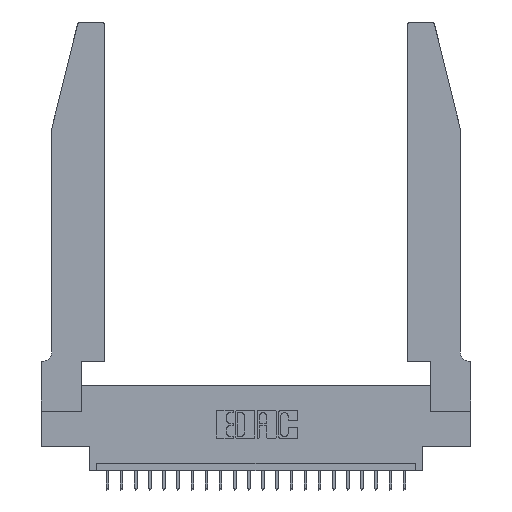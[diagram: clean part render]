
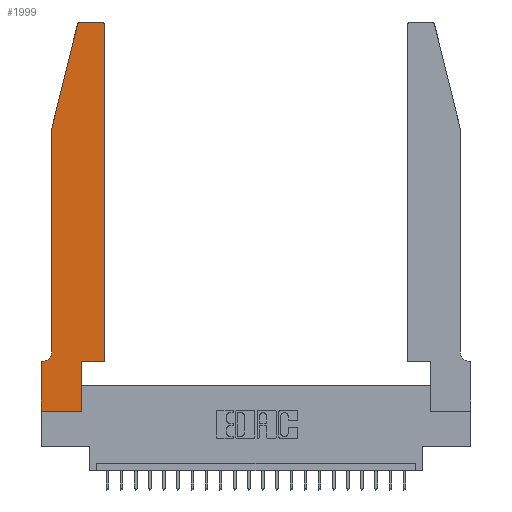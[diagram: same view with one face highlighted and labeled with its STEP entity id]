
A CAD part, top view. The second image highlights one B-rep face of the part: STEP entity #1999.
In plain terms, the highlighted planar face has unit normal (0, 0, 1).
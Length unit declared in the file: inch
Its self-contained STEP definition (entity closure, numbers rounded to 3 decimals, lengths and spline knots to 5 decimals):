
#53 = EDGE_CURVE ( 'NONE', #19041, #15948, #1308, .T. ) ;
#286 = ORIENTED_EDGE ( 'NONE', *, *, #4977, .T. ) ;
#426 = DIRECTION ( 'NONE',  ( -0.239, -0.971, 0. ) ) ;
#680 = ORIENTED_EDGE ( 'NONE', *, *, #19117, .T. ) ;
#777 = VECTOR ( 'NONE', #14901, 39.37008 ) ;
#782 = AXIS2_PLACEMENT_3D ( 'NONE', #13090, #3987, #14873 ) ;
#1308 = LINE ( 'NONE', #12774, #8461 ) ;
#1507 = ORIENTED_EDGE ( 'NONE', *, *, #4886, .T. ) ;
#1548 = VERTEX_POINT ( 'NONE', #2084 ) ;
#1744 = DIRECTION ( 'NONE',  ( 0., -1., 0. ) ) ;
#1999 = ADVANCED_FACE ( 'NONE', ( #22754 ), #20563, .T. ) ;
#2084 = CARTESIAN_POINT ( 'NONE',  ( 0.0755, 0.42, 0.37 ) ) ;
#2212 = EDGE_CURVE ( 'NONE', #3683, #22415, #21882, .T. ) ;
#2491 = DIRECTION ( 'NONE',  ( -1., 0., 0. ) ) ;
#2738 = EDGE_CURVE ( 'NONE', #4874, #9804, #19189, .T. ) ;
#3295 = CARTESIAN_POINT ( 'NONE',  ( 0.4205, 2.75, 0.37 ) ) ;
#3527 = CARTESIAN_POINT ( 'NONE',  ( 0., 0.35, 0.37 ) ) ;
#3683 = VERTEX_POINT ( 'NONE', #18636 ) ;
#3987 = DIRECTION ( 'NONE',  ( 0., 0., 1. ) ) ;
#4352 = CARTESIAN_POINT ( 'NONE',  ( 0.4505, 0.35, 0.37 ) ) ;
#4536 = CIRCLE ( 'NONE', #10803, 0.03 ) ;
#4874 = VERTEX_POINT ( 'NONE', #17412 ) ;
#4886 = EDGE_CURVE ( 'NONE', #22457, #3683, #23874, .T. ) ;
#4977 = EDGE_CURVE ( 'NONE', #16996, #4874, #4536, .T. ) ;
#5588 = CARTESIAN_POINT ( 'NONE',  ( 0., 0., 0.37 ) ) ;
#5748 = CARTESIAN_POINT ( 'NONE',  ( 0.0055, 0.42, 0.37 ) ) ;
#6837 = VERTEX_POINT ( 'NONE', #9846 ) ;
#7290 = CARTESIAN_POINT ( 'NONE',  ( 0., 0., 0.37 ) ) ;
#7775 = EDGE_CURVE ( 'NONE', #23308, #16996, #15610, .T. ) ;
#8461 = VECTOR ( 'NONE', #10922, 39.37008 ) ;
#8566 = CARTESIAN_POINT ( 'NONE',  ( 0., 0.35, 0.37 ) ) ;
#8638 = EDGE_CURVE ( 'NONE', #9804, #1548, #14750, .T. ) ;
#9295 = DIRECTION ( 'NONE',  ( 0., -1., 0. ) ) ;
#9340 = ORIENTED_EDGE ( 'NONE', *, *, #14296, .T. ) ;
#9355 = DIRECTION ( 'NONE',  ( -1., 0., 0. ) ) ;
#9476 = DIRECTION ( 'NONE',  ( 1., 0., 0. ) ) ;
#9804 = VERTEX_POINT ( 'NONE', #13866 ) ;
#9846 = CARTESIAN_POINT ( 'NONE',  ( 0.4505, 2.72, 0.37 ) ) ;
#10591 = DIRECTION ( 'NONE',  ( 0., 1., 0. ) ) ;
#10730 = ORIENTED_EDGE ( 'NONE', *, *, #16136, .T. ) ;
#10803 = AXIS2_PLACEMENT_3D ( 'NONE', #20234, #22051, #9476 ) ;
#10891 = CARTESIAN_POINT ( 'NONE',  ( 0.4505, 0.35, 0.37 ) ) ;
#10922 = DIRECTION ( 'NONE',  ( -1., 0., 0. ) ) ;
#11099 = CARTESIAN_POINT ( 'NONE',  ( 0.2865, 0., 0.37 ) ) ;
#11759 = CARTESIAN_POINT ( 'NONE',  ( 0.0755, 2., 0.37 ) ) ;
#11798 = CIRCLE ( 'NONE', #782, 0.03 ) ;
#11854 = DIRECTION ( 'NONE',  ( 0., 1., 0. ) ) ;
#12710 = CARTESIAN_POINT ( 'NONE',  ( 0.4505, 0.35, 0.37 ) ) ;
#12736 = VECTOR ( 'NONE', #11854, 39.37008 ) ;
#12774 = CARTESIAN_POINT ( 'NONE',  ( 0.0755, 0.35, 0.37 ) ) ;
#12817 = VECTOR ( 'NONE', #1744, 39.37008 ) ;
#13029 = DIRECTION ( 'NONE',  ( 0., 0., -1. ) ) ;
#13090 = CARTESIAN_POINT ( 'NONE',  ( 0.4205, 2.72, 0.37 ) ) ;
#13116 = CARTESIAN_POINT ( 'NONE',  ( 0., 0., 0.37 ) ) ;
#13446 = CARTESIAN_POINT ( 'NONE',  ( 0.284, 2.75, 0.37 ) ) ;
#13663 = ORIENTED_EDGE ( 'NONE', *, *, #53, .T. ) ;
#13866 = CARTESIAN_POINT ( 'NONE',  ( 0.0755, 2., 0.37 ) ) ;
#14010 = CARTESIAN_POINT ( 'NONE',  ( 0.2865, 0.35, 0.37 ) ) ;
#14296 = EDGE_CURVE ( 'NONE', #1548, #19041, #17600, .T. ) ;
#14462 = ORIENTED_EDGE ( 'NONE', *, *, #8638, .T. ) ;
#14750 = LINE ( 'NONE', #18526, #12817 ) ;
#14821 = EDGE_CURVE ( 'NONE', #6837, #23308, #11798, .T. ) ;
#14870 = VECTOR ( 'NONE', #9295, 39.37008 ) ;
#14873 = DIRECTION ( 'NONE',  ( 1., 0., 0. ) ) ;
#14901 = DIRECTION ( 'NONE',  ( 1., 0., 0. ) ) ;
#14988 = ORIENTED_EDGE ( 'NONE', *, *, #23970, .T. ) ;
#15597 = VERTEX_POINT ( 'NONE', #5588 ) ;
#15604 = LINE ( 'NONE', #4352, #12736 ) ;
#15610 = LINE ( 'NONE', #17315, #17453 ) ;
#15948 = VERTEX_POINT ( 'NONE', #8566 ) ;
#16100 = ORIENTED_EDGE ( 'NONE', *, *, #14821, .T. ) ;
#16136 = EDGE_CURVE ( 'NONE', #15948, #15597, #24059, .T. ) ;
#16996 = VERTEX_POINT ( 'NONE', #13446 ) ;
#17315 = CARTESIAN_POINT ( 'NONE',  ( 0.2605, 2.75, 0.37 ) ) ;
#17412 = CARTESIAN_POINT ( 'NONE',  ( 0.25487, 2.72718, 0.37 ) ) ;
#17453 = VECTOR ( 'NONE', #2491, 39.37008 ) ;
#17600 = CIRCLE ( 'NONE', #22682, 0.07 ) ;
#18313 = DIRECTION ( 'NONE',  ( 1., 0., 0. ) ) ;
#18517 = AXIS2_PLACEMENT_3D ( 'NONE', #3527, #22511, #18833 ) ;
#18526 = CARTESIAN_POINT ( 'NONE',  ( 0.0755, 2., 0.37 ) ) ;
#18537 = VECTOR ( 'NONE', #10591, 39.37008 ) ;
#18611 = ORIENTED_EDGE ( 'NONE', *, *, #2738, .T. ) ;
#18636 = CARTESIAN_POINT ( 'NONE',  ( 0.2865, 0.35, 0.37 ) ) ;
#18833 = DIRECTION ( 'NONE',  ( 1., 0., 0. ) ) ;
#19041 = VERTEX_POINT ( 'NONE', #21793 ) ;
#19117 = EDGE_CURVE ( 'NONE', #15597, #22457, #20796, .T. ) ;
#19189 = LINE ( 'NONE', #11759, #20356 ) ;
#19518 = ORIENTED_EDGE ( 'NONE', *, *, #7775, .T. ) ;
#20234 = CARTESIAN_POINT ( 'NONE',  ( 0.284, 2.72, 0.37 ) ) ;
#20356 = VECTOR ( 'NONE', #426, 39.37008 ) ;
#20563 = PLANE ( 'NONE',  #18517 ) ;
#20796 = LINE ( 'NONE', #13116, #777 ) ;
#21793 = CARTESIAN_POINT ( 'NONE',  ( 0.0055, 0.35, 0.37 ) ) ;
#21882 = LINE ( 'NONE', #10891, #23907 ) ;
#22051 = DIRECTION ( 'NONE',  ( 0., 0., 1. ) ) ;
#22415 = VERTEX_POINT ( 'NONE', #12710 ) ;
#22457 = VERTEX_POINT ( 'NONE', #11099 ) ;
#22511 = DIRECTION ( 'NONE',  ( 0., 0., 1. ) ) ;
#22513 = ORIENTED_EDGE ( 'NONE', *, *, #2212, .T. ) ;
#22682 = AXIS2_PLACEMENT_3D ( 'NONE', #5748, #13029, #9355 ) ;
#22754 = FACE_OUTER_BOUND ( 'NONE', #23639, .T. ) ;
#23308 = VERTEX_POINT ( 'NONE', #3295 ) ;
#23639 = EDGE_LOOP ( 'NONE', ( #19518, #286, #18611, #14462, #9340, #13663, #10730, #680, #1507, #22513, #14988, #16100 ) ) ;
#23874 = LINE ( 'NONE', #14010, #18537 ) ;
#23907 = VECTOR ( 'NONE', #18313, 39.37008 ) ;
#23970 = EDGE_CURVE ( 'NONE', #22415, #6837, #15604, .T. ) ;
#24059 = LINE ( 'NONE', #7290, #14870 ) ;
